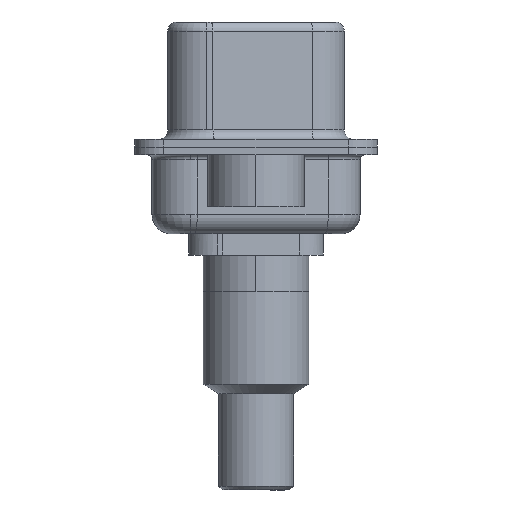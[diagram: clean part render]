
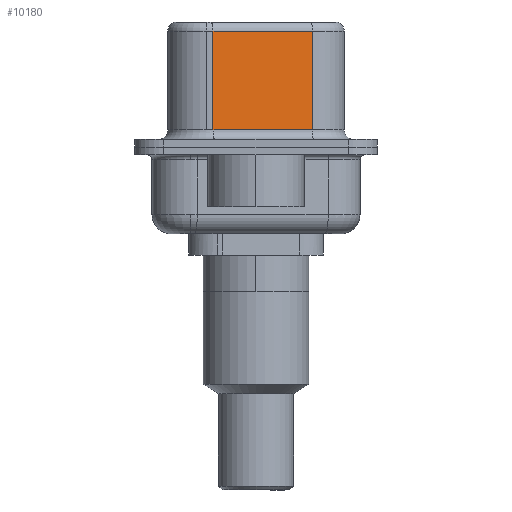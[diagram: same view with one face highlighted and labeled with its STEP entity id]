
A CAD part, left-side view. The second image highlights one B-rep face of the part: STEP entity #10180.
In plain terms, the highlighted planar face has unit normal (-0.985, -0.174, 0).
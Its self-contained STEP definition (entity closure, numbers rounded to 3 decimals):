
#863 = DIRECTION ( 'NONE',  ( 0., 0., -1. ) ) ;
#2738 = ORIENTED_EDGE ( 'NONE', *, *, #13999, .T. ) ;
#2897 = VECTOR ( 'NONE', #863, 1000. ) ;
#2931 = VECTOR ( 'NONE', #12622, 1000. ) ;
#3203 = CARTESIAN_POINT ( 'NONE',  ( 4.585, -2.927, 0.9 ) ) ;
#3426 = CARTESIAN_POINT ( 'NONE',  ( 3.675, 2.233, 6.52 ) ) ;
#3577 = EDGE_CURVE ( 'NONE', #13222, #16747, #17587, .T. ) ;
#3878 = EDGE_CURVE ( 'NONE', #19838, #13222, #4790, .T. ) ;
#4699 = EDGE_LOOP ( 'NONE', ( #10284, #5382, #11583, #2738 ) ) ;
#4790 = LINE ( 'NONE', #19879, #9511 ) ;
#5382 = ORIENTED_EDGE ( 'NONE', *, *, #3878, .T. ) ;
#5999 = CARTESIAN_POINT ( 'NONE',  ( 4.585, -2.927, 0.9 ) ) ;
#6382 = DIRECTION ( 'NONE',  ( 0.985, 0.174, 0. ) ) ;
#7112 = LINE ( 'NONE', #3203, #2931 ) ;
#7888 = PLANE ( 'NONE',  #13756 ) ;
#8136 = DIRECTION ( 'NONE',  ( -0.174, 0.985, 0. ) ) ;
#8643 = CARTESIAN_POINT ( 'NONE',  ( 4.585, -2.927, 6.52 ) ) ;
#8696 = CARTESIAN_POINT ( 'NONE',  ( 4.585, -2.927, 6.02 ) ) ;
#9511 = VECTOR ( 'NONE', #8136, 1000. ) ;
#10180 = ADVANCED_FACE ( 'NONE', ( #16224 ), #7888, .F. ) ;
#10284 = ORIENTED_EDGE ( 'NONE', *, *, #15577, .F. ) ;
#11583 = ORIENTED_EDGE ( 'NONE', *, *, #3577, .T. ) ;
#12622 = DIRECTION ( 'NONE',  ( 0.174, -0.985, 0. ) ) ;
#12781 = CARTESIAN_POINT ( 'NONE',  ( 3.675, 2.233, 6.02 ) ) ;
#13222 = VERTEX_POINT ( 'NONE', #12781 ) ;
#13756 = AXIS2_PLACEMENT_3D ( 'NONE', #15765, #6382, #17327 ) ;
#13999 = EDGE_CURVE ( 'NONE', #16747, #14938, #7112, .T. ) ;
#14938 = VERTEX_POINT ( 'NONE', #5999 ) ;
#15393 = LINE ( 'NONE', #8643, #2897 ) ;
#15577 = EDGE_CURVE ( 'NONE', #19838, #14938, #15393, .T. ) ;
#15765 = CARTESIAN_POINT ( 'NONE',  ( 4.585, -2.927, 6.52 ) ) ;
#16196 = CARTESIAN_POINT ( 'NONE',  ( 3.675, 2.233, 0.9 ) ) ;
#16224 = FACE_OUTER_BOUND ( 'NONE', #4699, .T. ) ;
#16747 = VERTEX_POINT ( 'NONE', #16196 ) ;
#17094 = VECTOR ( 'NONE', #17540, 1000. ) ;
#17327 = DIRECTION ( 'NONE',  ( -0.174, 0.985, 0. ) ) ;
#17540 = DIRECTION ( 'NONE',  ( 0., 0., -1. ) ) ;
#17587 = LINE ( 'NONE', #3426, #17094 ) ;
#19838 = VERTEX_POINT ( 'NONE', #8696 ) ;
#19879 = CARTESIAN_POINT ( 'NONE',  ( 4.585, -2.927, 6.02 ) ) ;
